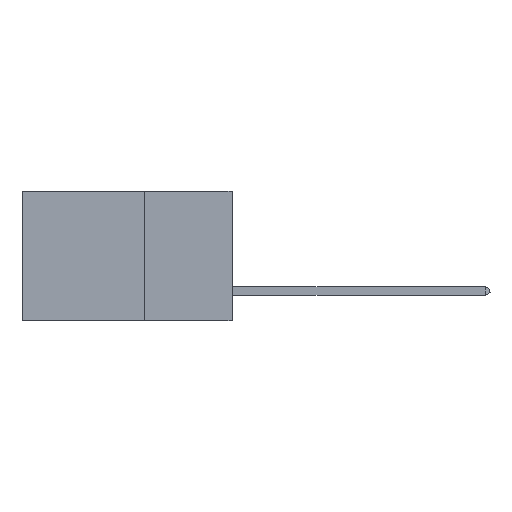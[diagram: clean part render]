
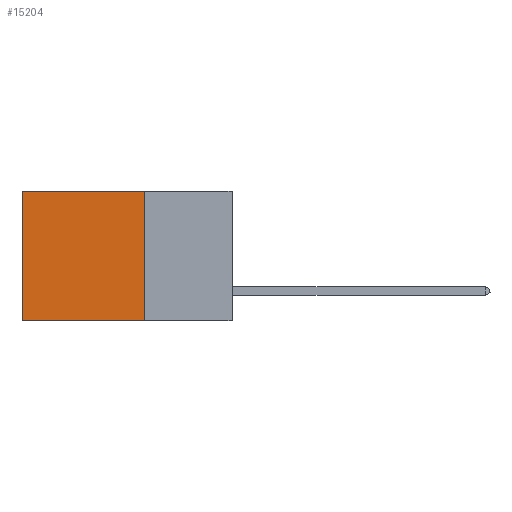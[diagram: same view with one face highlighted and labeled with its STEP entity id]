
A CAD part, left-side view. The second image highlights one B-rep face of the part: STEP entity #15204.
In plain terms, the highlighted planar face has unit normal (-1, 0, 0).
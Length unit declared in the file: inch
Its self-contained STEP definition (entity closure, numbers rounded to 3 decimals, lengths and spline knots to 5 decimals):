
#291 = EDGE_CURVE ( 'NONE', #12508, #14494, #17303, .T. ) ;
#1430 = CARTESIAN_POINT ( 'NONE',  ( 0.2875, 0.25, -0.37 ) ) ;
#1493 = VERTEX_POINT ( 'NONE', #7008 ) ;
#1589 = VECTOR ( 'NONE', #19260, 39.37008 ) ;
#1735 = LINE ( 'NONE', #9519, #4913 ) ;
#2799 = DIRECTION ( 'NONE',  ( 0., 0., -1. ) ) ;
#3132 = VECTOR ( 'NONE', #21730, 39.37008 ) ;
#3186 = DIRECTION ( 'NONE',  ( 0., 0., -1. ) ) ;
#4544 = ORIENTED_EDGE ( 'NONE', *, *, #291, .T. ) ;
#4913 = VECTOR ( 'NONE', #2799, 39.37008 ) ;
#5768 = ORIENTED_EDGE ( 'NONE', *, *, #15656, .F. ) ;
#5878 = CARTESIAN_POINT ( 'NONE',  ( 0.2875, 0.6, 0. ) ) ;
#6218 = CARTESIAN_POINT ( 'NONE',  ( 0.2875, 0.25, 0. ) ) ;
#6841 = CARTESIAN_POINT ( 'NONE',  ( 0.2875, 0.25, -0.37 ) ) ;
#7008 = CARTESIAN_POINT ( 'NONE',  ( 0.2875, 0.6, -0.37 ) ) ;
#8900 = EDGE_LOOP ( 'NONE', ( #12738, #9322, #5768, #4544 ) ) ;
#9283 = CARTESIAN_POINT ( 'NONE',  ( 0.2875, 0.6, 0. ) ) ;
#9322 = ORIENTED_EDGE ( 'NONE', *, *, #15201, .F. ) ;
#9519 = CARTESIAN_POINT ( 'NONE',  ( 0.2875, 0.25, 0. ) ) ;
#9705 = FACE_OUTER_BOUND ( 'NONE', #8900, .T. ) ;
#10019 = LINE ( 'NONE', #5878, #1589 ) ;
#12508 = VERTEX_POINT ( 'NONE', #18011 ) ;
#12738 = ORIENTED_EDGE ( 'NONE', *, *, #20416, .T. ) ;
#13036 = PLANE ( 'NONE',  #14248 ) ;
#13225 = VERTEX_POINT ( 'NONE', #6841 ) ;
#13339 = LINE ( 'NONE', #1430, #20919 ) ;
#14248 = AXIS2_PLACEMENT_3D ( 'NONE', #21598, #18164, #3186 ) ;
#14494 = VERTEX_POINT ( 'NONE', #9283 ) ;
#14771 = DIRECTION ( 'NONE',  ( 0., 1., 0. ) ) ;
#15201 = EDGE_CURVE ( 'NONE', #13225, #1493, #13339, .T. ) ;
#15204 = ADVANCED_FACE ( 'NONE', ( #9705 ), #13036, .F. ) ;
#15656 = EDGE_CURVE ( 'NONE', #12508, #13225, #1735, .T. ) ;
#17303 = LINE ( 'NONE', #6218, #3132 ) ;
#18011 = CARTESIAN_POINT ( 'NONE',  ( 0.2875, 0.25, 0. ) ) ;
#18164 = DIRECTION ( 'NONE',  ( 1., 0., 0. ) ) ;
#19260 = DIRECTION ( 'NONE',  ( 0., 0., -1. ) ) ;
#20416 = EDGE_CURVE ( 'NONE', #14494, #1493, #10019, .T. ) ;
#20919 = VECTOR ( 'NONE', #14771, 39.37008 ) ;
#21598 = CARTESIAN_POINT ( 'NONE',  ( 0.2875, 0.25, 0. ) ) ;
#21730 = DIRECTION ( 'NONE',  ( 0., 1., 0. ) ) ;
